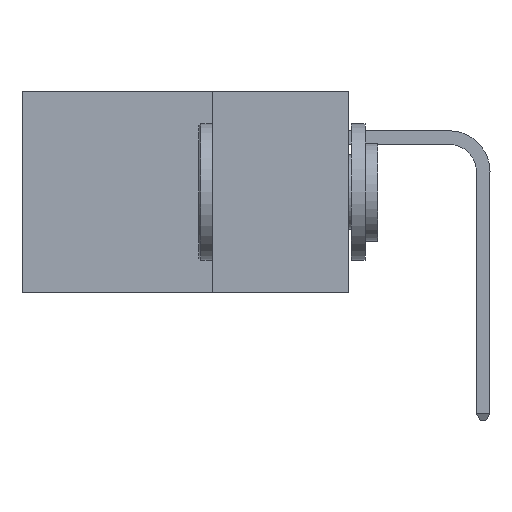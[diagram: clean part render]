
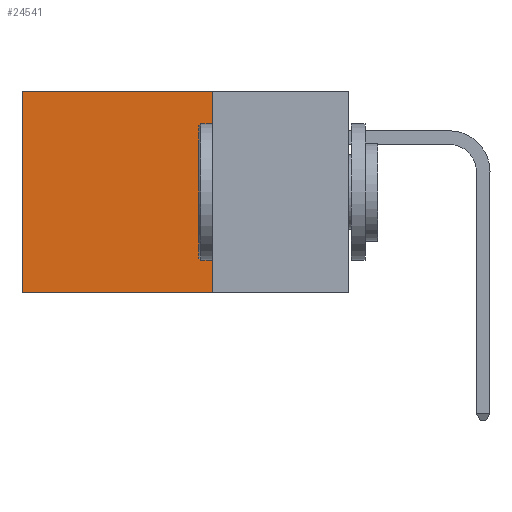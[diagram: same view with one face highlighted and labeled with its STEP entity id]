
A CAD part, left-side view. The second image highlights one B-rep face of the part: STEP entity #24541.
In plain terms, the highlighted planar face has unit normal (-1, 0, 0).
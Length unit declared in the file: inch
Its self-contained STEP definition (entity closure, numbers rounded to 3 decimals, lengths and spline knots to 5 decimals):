
#3610 = CARTESIAN_POINT ( 'NONE',  ( 0.2875, 0.6, 0. ) ) ;
#4768 = ORIENTED_EDGE ( 'NONE', *, *, #7393, .F. ) ;
#5376 = VECTOR ( 'NONE', #30426, 39.37008 ) ;
#5494 = VERTEX_POINT ( 'NONE', #3610 ) ;
#6065 = CARTESIAN_POINT ( 'NONE',  ( 0.2875, 0.25, 0. ) ) ;
#7044 = EDGE_CURVE ( 'NONE', #16638, #12251, #23745, .T. ) ;
#7393 = EDGE_CURVE ( 'NONE', #12251, #28543, #14464, .T. ) ;
#7751 = AXIS2_PLACEMENT_3D ( 'NONE', #8496, #35320, #17555 ) ;
#8496 = CARTESIAN_POINT ( 'NONE',  ( 0.2875, 0.25, 0. ) ) ;
#11411 = EDGE_LOOP ( 'NONE', ( #15830, #4768, #14898, #32591 ) ) ;
#12251 = VERTEX_POINT ( 'NONE', #23906 ) ;
#14230 = EDGE_CURVE ( 'NONE', #5494, #28543, #20346, .T. ) ;
#14464 = LINE ( 'NONE', #30576, #19615 ) ;
#14898 = ORIENTED_EDGE ( 'NONE', *, *, #7044, .F. ) ;
#15830 = ORIENTED_EDGE ( 'NONE', *, *, #14230, .T. ) ;
#16638 = VERTEX_POINT ( 'NONE', #6065 ) ;
#17417 = PLANE ( 'NONE',  #7751 ) ;
#17555 = DIRECTION ( 'NONE',  ( 0., 0., -1. ) ) ;
#18668 = CARTESIAN_POINT ( 'NONE',  ( 0.2875, 0.6, 0. ) ) ;
#19615 = VECTOR ( 'NONE', #33562, 39.37008 ) ;
#20346 = LINE ( 'NONE', #18668, #5376 ) ;
#20824 = LINE ( 'NONE', #34752, #26866 ) ;
#21091 = FACE_OUTER_BOUND ( 'NONE', #11411, .T. ) ;
#22875 = DIRECTION ( 'NONE',  ( 0., 1., 0. ) ) ;
#23745 = LINE ( 'NONE', #37465, #24680 ) ;
#23906 = CARTESIAN_POINT ( 'NONE',  ( 0.2875, 0.25, -0.37 ) ) ;
#24541 = ADVANCED_FACE ( 'NONE', ( #21091 ), #17417, .F. ) ;
#24680 = VECTOR ( 'NONE', #25649, 39.37008 ) ;
#25185 = CARTESIAN_POINT ( 'NONE',  ( 0.2875, 0.6, -0.37 ) ) ;
#25649 = DIRECTION ( 'NONE',  ( 0., 0., -1. ) ) ;
#26866 = VECTOR ( 'NONE', #22875, 39.37008 ) ;
#28543 = VERTEX_POINT ( 'NONE', #25185 ) ;
#30426 = DIRECTION ( 'NONE',  ( 0., 0., -1. ) ) ;
#30576 = CARTESIAN_POINT ( 'NONE',  ( 0.2875, 0.25, -0.37 ) ) ;
#31403 = EDGE_CURVE ( 'NONE', #16638, #5494, #20824, .T. ) ;
#32591 = ORIENTED_EDGE ( 'NONE', *, *, #31403, .T. ) ;
#33562 = DIRECTION ( 'NONE',  ( 0., 1., 0. ) ) ;
#34752 = CARTESIAN_POINT ( 'NONE',  ( 0.2875, 0.25, 0. ) ) ;
#35320 = DIRECTION ( 'NONE',  ( 1., 0., 0. ) ) ;
#37465 = CARTESIAN_POINT ( 'NONE',  ( 0.2875, 0.25, 0. ) ) ;
